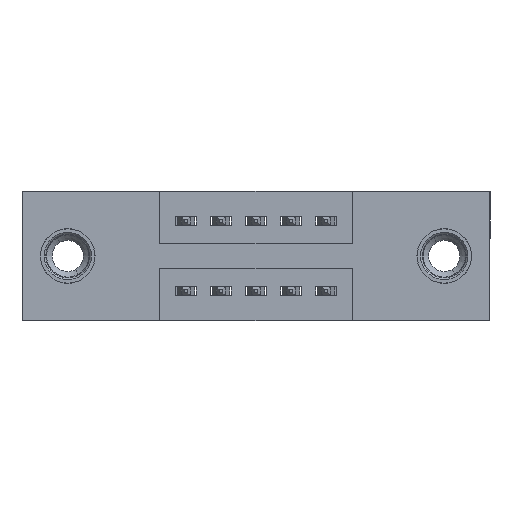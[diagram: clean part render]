
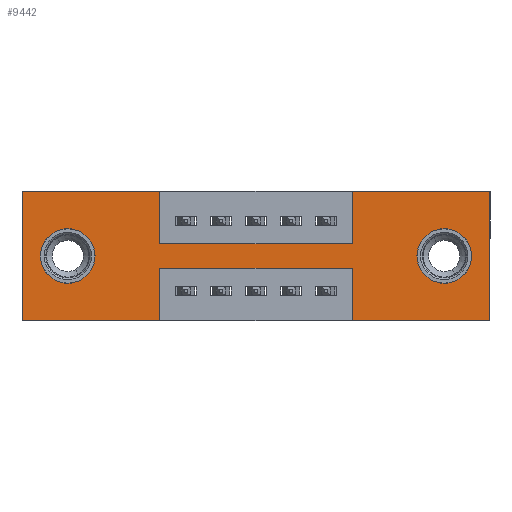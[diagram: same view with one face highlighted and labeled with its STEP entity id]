
A CAD part, front view. The second image highlights one B-rep face of the part: STEP entity #9442.
In plain terms, the highlighted planar face has unit normal (0, -1, 0).
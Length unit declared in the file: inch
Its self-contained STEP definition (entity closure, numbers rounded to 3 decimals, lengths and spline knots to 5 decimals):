
#16 = VERTEX_POINT ( 'NONE', #10278 ) ;
#64 = DIRECTION ( 'NONE',  ( 0., 0., 1. ) ) ;
#259 = CARTESIAN_POINT ( 'NONE',  ( 0.13, 0., -0.263 ) ) ;
#307 = VERTEX_POINT ( 'NONE', #10690 ) ;
#728 = AXIS2_PLACEMENT_3D ( 'NONE', #866, #9391, #9212 ) ;
#732 = LINE ( 'NONE', #10574, #11605 ) ;
#866 = CARTESIAN_POINT ( 'NONE',  ( 0.13, 0., -0.185 ) ) ;
#895 = PLANE ( 'NONE',  #5630 ) ;
#941 = EDGE_CURVE ( 'NONE', #8323, #307, #4903, .T. ) ;
#1173 = VERTEX_POINT ( 'NONE', #7982 ) ;
#1346 = VERTEX_POINT ( 'NONE', #12762 ) ;
#1496 = VECTOR ( 'NONE', #64, 39.37008 ) ;
#1658 = FACE_BOUND ( 'NONE', #11170, .T. ) ;
#1705 = DIRECTION ( 'NONE',  ( 0., 0., 1. ) ) ;
#1799 = ORIENTED_EDGE ( 'NONE', *, *, #8944, .F. ) ;
#1926 = EDGE_CURVE ( 'NONE', #2469, #2505, #5385, .T. ) ;
#2100 = VERTEX_POINT ( 'NONE', #10125 ) ;
#2121 = CARTESIAN_POINT ( 'NONE',  ( 0.3925, 0., -0.37 ) ) ;
#2258 = CARTESIAN_POINT ( 'NONE',  ( 0., 0., 0. ) ) ;
#2469 = VERTEX_POINT ( 'NONE', #10343 ) ;
#2505 = VERTEX_POINT ( 'NONE', #12618 ) ;
#2538 = CARTESIAN_POINT ( 'NONE',  ( 0., 0., -0.37 ) ) ;
#2606 = EDGE_LOOP ( 'NONE', ( #3371, #9657, #7308, #11112, #3538, #6619, #1799, #11735, #6240, #5722, #7376, #12272 ) ) ;
#2799 = EDGE_CURVE ( 'NONE', #10601, #2100, #11464, .T. ) ;
#2810 = EDGE_CURVE ( 'NONE', #6590, #4901, #9324, .T. ) ;
#2897 = EDGE_CURVE ( 'NONE', #307, #11322, #5710, .T. ) ;
#2993 = CARTESIAN_POINT ( 'NONE',  ( 0.3925, 0., -0.15 ) ) ;
#3024 = VECTOR ( 'NONE', #3373, 39.37008 ) ;
#3174 = EDGE_CURVE ( 'NONE', #8965, #16, #7498, .T. ) ;
#3287 = LINE ( 'NONE', #7578, #1496 ) ;
#3371 = ORIENTED_EDGE ( 'NONE', *, *, #6500, .F. ) ;
#3373 = DIRECTION ( 'NONE',  ( 1., 0., 0. ) ) ;
#3538 = ORIENTED_EDGE ( 'NONE', *, *, #7507, .F. ) ;
#3571 = VECTOR ( 'NONE', #8656, 39.37008 ) ;
#3588 = DIRECTION ( 'NONE',  ( -1., 0., 0. ) ) ;
#4277 = FACE_BOUND ( 'NONE', #6502, .T. ) ;
#4457 = VECTOR ( 'NONE', #6487, 39.37008 ) ;
#4646 = VECTOR ( 'NONE', #9190, 39.37008 ) ;
#4722 = CARTESIAN_POINT ( 'NONE',  ( 0.13, 0., -0.185 ) ) ;
#4773 = DIRECTION ( 'NONE',  ( 0., 0., 1. ) ) ;
#4901 = VERTEX_POINT ( 'NONE', #13029 ) ;
#4903 = LINE ( 'NONE', #2538, #9525 ) ;
#4964 = ORIENTED_EDGE ( 'NONE', *, *, #2799, .T. ) ;
#4997 = CARTESIAN_POINT ( 'NONE',  ( 1.205, 0., -0.185 ) ) ;
#5140 = DIRECTION ( 'NONE',  ( -1., 0., 0. ) ) ;
#5285 = VERTEX_POINT ( 'NONE', #7334 ) ;
#5385 = LINE ( 'NONE', #5430, #3571 ) ;
#5430 = CARTESIAN_POINT ( 'NONE',  ( 0.3925, 0., 0. ) ) ;
#5630 = AXIS2_PLACEMENT_3D ( 'NONE', #13451, #7095, #10337 ) ;
#5710 = LINE ( 'NONE', #12540, #9168 ) ;
#5722 = ORIENTED_EDGE ( 'NONE', *, *, #13422, .F. ) ;
#5857 = ORIENTED_EDGE ( 'NONE', *, *, #8608, .T. ) ;
#5994 = CIRCLE ( 'NONE', #6535, 0.078 ) ;
#6053 = CARTESIAN_POINT ( 'NONE',  ( 0., 0., 0. ) ) ;
#6240 = ORIENTED_EDGE ( 'NONE', *, *, #1926, .F. ) ;
#6323 = VECTOR ( 'NONE', #5140, 39.37008 ) ;
#6487 = DIRECTION ( 'NONE',  ( -1., 0., 0. ) ) ;
#6500 = EDGE_CURVE ( 'NONE', #1173, #8323, #732, .T. ) ;
#6502 = EDGE_LOOP ( 'NONE', ( #5857, #13067 ) ) ;
#6519 = VECTOR ( 'NONE', #1705, 39.37008 ) ;
#6535 = AXIS2_PLACEMENT_3D ( 'NONE', #12764, #8549, #12724 ) ;
#6590 = VERTEX_POINT ( 'NONE', #6976 ) ;
#6619 = ORIENTED_EDGE ( 'NONE', *, *, #12478, .F. ) ;
#6754 = CARTESIAN_POINT ( 'NONE',  ( 0.9425, 0., -0.37 ) ) ;
#6912 = DIRECTION ( 'NONE',  ( 0., 0., -1. ) ) ;
#6976 = CARTESIAN_POINT ( 'NONE',  ( 0.9425, 0., -0.37 ) ) ;
#6978 = DIRECTION ( 'NONE',  ( 0., 1., 0. ) ) ;
#7089 = CIRCLE ( 'NONE', #11540, 0.078 ) ;
#7095 = DIRECTION ( 'NONE',  ( 0., -1., 0. ) ) ;
#7257 = CARTESIAN_POINT ( 'NONE',  ( 0.9425, 0., -0.15 ) ) ;
#7304 = LINE ( 'NONE', #8636, #3024 ) ;
#7308 = ORIENTED_EDGE ( 'NONE', *, *, #2810, .F. ) ;
#7334 = CARTESIAN_POINT ( 'NONE',  ( 0.9425, 0., 0. ) ) ;
#7376 = ORIENTED_EDGE ( 'NONE', *, *, #2897, .F. ) ;
#7381 = DIRECTION ( 'NONE',  ( 0., 0., -1. ) ) ;
#7454 = LINE ( 'NONE', #8206, #8613 ) ;
#7498 = CIRCLE ( 'NONE', #728, 0.078 ) ;
#7507 = EDGE_CURVE ( 'NONE', #7710, #1346, #7454, .T. ) ;
#7578 = CARTESIAN_POINT ( 'NONE',  ( 0.9425, 0., 0. ) ) ;
#7710 = VERTEX_POINT ( 'NONE', #11535 ) ;
#7982 = CARTESIAN_POINT ( 'NONE',  ( 0.3925, 0., -0.22 ) ) ;
#8178 = DIRECTION ( 'NONE',  ( 0., 0., 1. ) ) ;
#8206 = CARTESIAN_POINT ( 'NONE',  ( 1.335, 0., 0. ) ) ;
#8246 = LINE ( 'NONE', #8520, #4457 ) ;
#8313 = CARTESIAN_POINT ( 'NONE',  ( 0.3925, 0., -0.22 ) ) ;
#8323 = VERTEX_POINT ( 'NONE', #2121 ) ;
#8461 = EDGE_CURVE ( 'NONE', #1346, #6590, #8246, .T. ) ;
#8520 = CARTESIAN_POINT ( 'NONE',  ( 0., 0., -0.37 ) ) ;
#8549 = DIRECTION ( 'NONE',  ( 0., 1., 0. ) ) ;
#8608 = EDGE_CURVE ( 'NONE', #16, #8965, #7089, .T. ) ;
#8613 = VECTOR ( 'NONE', #6912, 39.37008 ) ;
#8636 = CARTESIAN_POINT ( 'NONE',  ( 0., 0., 0. ) ) ;
#8656 = DIRECTION ( 'NONE',  ( 0., 0., -1. ) ) ;
#8907 = VERTEX_POINT ( 'NONE', #7257 ) ;
#8944 = EDGE_CURVE ( 'NONE', #8907, #5285, #3287, .T. ) ;
#8965 = VERTEX_POINT ( 'NONE', #259 ) ;
#9107 = CARTESIAN_POINT ( 'NONE',  ( 1.205, 0., -0.107 ) ) ;
#9168 = VECTOR ( 'NONE', #8178, 39.37008 ) ;
#9190 = DIRECTION ( 'NONE',  ( 1., 0., 0. ) ) ;
#9212 = DIRECTION ( 'NONE',  ( 0., 0., 1. ) ) ;
#9324 = LINE ( 'NONE', #6754, #6519 ) ;
#9391 = DIRECTION ( 'NONE',  ( 0., 1., 0. ) ) ;
#9442 = ADVANCED_FACE ( 'NONE', ( #1658, #4277, #10213 ), #895, .T. ) ;
#9488 = DIRECTION ( 'NONE',  ( 1., 0., 0. ) ) ;
#9525 = VECTOR ( 'NONE', #3588, 39.37008 ) ;
#9657 = ORIENTED_EDGE ( 'NONE', *, *, #13008, .F. ) ;
#10125 = CARTESIAN_POINT ( 'NONE',  ( 1.205, 0., -0.263 ) ) ;
#10213 = FACE_OUTER_BOUND ( 'NONE', #2606, .T. ) ;
#10278 = CARTESIAN_POINT ( 'NONE',  ( 0.13, 0., -0.107 ) ) ;
#10337 = DIRECTION ( 'NONE',  ( 0., 0., -1. ) ) ;
#10343 = CARTESIAN_POINT ( 'NONE',  ( 0.3925, 0., 0. ) ) ;
#10574 = CARTESIAN_POINT ( 'NONE',  ( 0.3925, 0., -0.37 ) ) ;
#10601 = VERTEX_POINT ( 'NONE', #9107 ) ;
#10690 = CARTESIAN_POINT ( 'NONE',  ( 0., 0., -0.37 ) ) ;
#10894 = ORIENTED_EDGE ( 'NONE', *, *, #13169, .T. ) ;
#11112 = ORIENTED_EDGE ( 'NONE', *, *, #8461, .F. ) ;
#11170 = EDGE_LOOP ( 'NONE', ( #4964, #10894 ) ) ;
#11252 = DIRECTION ( 'NONE',  ( 0., 0., -1. ) ) ;
#11322 = VERTEX_POINT ( 'NONE', #2258 ) ;
#11464 = CIRCLE ( 'NONE', #11475, 0.078 ) ;
#11475 = AXIS2_PLACEMENT_3D ( 'NONE', #4997, #6978, #11252 ) ;
#11535 = CARTESIAN_POINT ( 'NONE',  ( 1.335, 0., 0. ) ) ;
#11540 = AXIS2_PLACEMENT_3D ( 'NONE', #4722, #12112, #4773 ) ;
#11605 = VECTOR ( 'NONE', #7381, 39.37008 ) ;
#11735 = ORIENTED_EDGE ( 'NONE', *, *, #12625, .F. ) ;
#11768 = LINE ( 'NONE', #8313, #6323 ) ;
#12112 = DIRECTION ( 'NONE',  ( 0., 1., 0. ) ) ;
#12272 = ORIENTED_EDGE ( 'NONE', *, *, #941, .F. ) ;
#12441 = VECTOR ( 'NONE', #9488, 39.37008 ) ;
#12478 = EDGE_CURVE ( 'NONE', #5285, #7710, #7304, .T. ) ;
#12540 = CARTESIAN_POINT ( 'NONE',  ( 0., 0., 0. ) ) ;
#12618 = CARTESIAN_POINT ( 'NONE',  ( 0.3925, 0., -0.15 ) ) ;
#12625 = EDGE_CURVE ( 'NONE', #2505, #8907, #13445, .T. ) ;
#12724 = DIRECTION ( 'NONE',  ( 0., 0., -1. ) ) ;
#12762 = CARTESIAN_POINT ( 'NONE',  ( 1.335, 0., -0.37 ) ) ;
#12764 = CARTESIAN_POINT ( 'NONE',  ( 1.205, 0., -0.185 ) ) ;
#12929 = LINE ( 'NONE', #6053, #4646 ) ;
#13008 = EDGE_CURVE ( 'NONE', #4901, #1173, #11768, .T. ) ;
#13029 = CARTESIAN_POINT ( 'NONE',  ( 0.9425, 0., -0.22 ) ) ;
#13067 = ORIENTED_EDGE ( 'NONE', *, *, #3174, .T. ) ;
#13169 = EDGE_CURVE ( 'NONE', #2100, #10601, #5994, .T. ) ;
#13422 = EDGE_CURVE ( 'NONE', #11322, #2469, #12929, .T. ) ;
#13445 = LINE ( 'NONE', #2993, #12441 ) ;
#13451 = CARTESIAN_POINT ( 'NONE',  ( 0., 0., -0.37 ) ) ;
